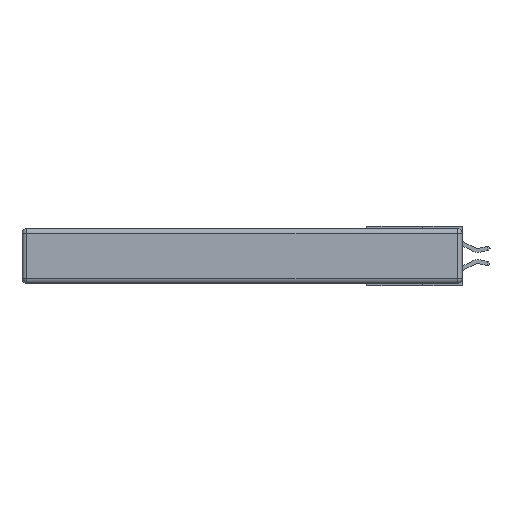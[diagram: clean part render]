
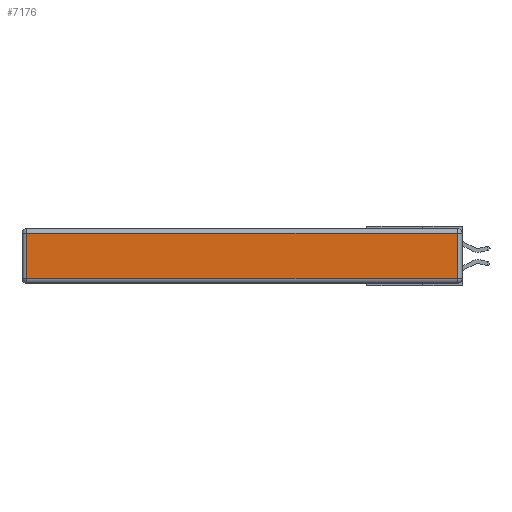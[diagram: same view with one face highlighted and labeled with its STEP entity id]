
A CAD part, left-side view. The second image highlights one B-rep face of the part: STEP entity #7176.
In plain terms, the highlighted planar face has unit normal (-1, 0, 0).
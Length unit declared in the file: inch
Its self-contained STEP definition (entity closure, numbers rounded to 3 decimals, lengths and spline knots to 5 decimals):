
#167 = ORIENTED_EDGE ( 'NONE', *, *, #7097, .T. ) ;
#291 = VERTEX_POINT ( 'NONE', #6391 ) ;
#1732 = CARTESIAN_POINT ( 'NONE',  ( 0., 2.72, -0.313 ) ) ;
#2081 = CARTESIAN_POINT ( 'NONE',  ( 0., 0.03, -0.343 ) ) ;
#2171 = AXIS2_PLACEMENT_3D ( 'NONE', #10414, #3693, #8972 ) ;
#2282 = CARTESIAN_POINT ( 'NONE',  ( 0., 0.03, -0.313 ) ) ;
#2345 = CARTESIAN_POINT ( 'NONE',  ( 0., 2.72, -0.343 ) ) ;
#3225 = VECTOR ( 'NONE', #9730, 39.37008 ) ;
#3486 = DIRECTION ( 'NONE',  ( 0., 0., -1. ) ) ;
#3516 = VECTOR ( 'NONE', #10558, 39.37008 ) ;
#3693 = DIRECTION ( 'NONE',  ( -1., 0., 0. ) ) ;
#4146 = EDGE_CURVE ( 'NONE', #11135, #291, #5779, .T. ) ;
#4260 = EDGE_CURVE ( 'NONE', #291, #5105, #10240, .T. ) ;
#4977 = ORIENTED_EDGE ( 'NONE', *, *, #11480, .T. ) ;
#5105 = VERTEX_POINT ( 'NONE', #11224 ) ;
#5412 = FACE_OUTER_BOUND ( 'NONE', #10138, .T. ) ;
#5779 = LINE ( 'NONE', #2081, #3225 ) ;
#6391 = CARTESIAN_POINT ( 'NONE',  ( 0., 0.03, -0.03 ) ) ;
#7048 = LINE ( 'NONE', #2345, #11525 ) ;
#7097 = EDGE_CURVE ( 'NONE', #5105, #11298, #7048, .T. ) ;
#7176 = ADVANCED_FACE ( 'NONE', ( #5412 ), #9408, .T. ) ;
#7203 = LINE ( 'NONE', #8542, #11667 ) ;
#7601 = ORIENTED_EDGE ( 'NONE', *, *, #4146, .T. ) ;
#8332 = ORIENTED_EDGE ( 'NONE', *, *, #4260, .T. ) ;
#8542 = CARTESIAN_POINT ( 'NONE',  ( 0., 0., -0.313 ) ) ;
#8705 = CARTESIAN_POINT ( 'NONE',  ( 0., 2.75, -0.03 ) ) ;
#8972 = DIRECTION ( 'NONE',  ( 0., 0., 1. ) ) ;
#9408 = PLANE ( 'NONE',  #2171 ) ;
#9730 = DIRECTION ( 'NONE',  ( 0., 0., 1. ) ) ;
#10138 = EDGE_LOOP ( 'NONE', ( #4977, #7601, #8332, #167 ) ) ;
#10240 = LINE ( 'NONE', #8705, #3516 ) ;
#10414 = CARTESIAN_POINT ( 'NONE',  ( 0., 0., -0.343 ) ) ;
#10558 = DIRECTION ( 'NONE',  ( 0., 1., 0. ) ) ;
#11135 = VERTEX_POINT ( 'NONE', #2282 ) ;
#11224 = CARTESIAN_POINT ( 'NONE',  ( 0., 2.72, -0.03 ) ) ;
#11298 = VERTEX_POINT ( 'NONE', #1732 ) ;
#11308 = DIRECTION ( 'NONE',  ( 0., -1., 0. ) ) ;
#11480 = EDGE_CURVE ( 'NONE', #11298, #11135, #7203, .T. ) ;
#11525 = VECTOR ( 'NONE', #3486, 39.37008 ) ;
#11667 = VECTOR ( 'NONE', #11308, 39.37008 ) ;
